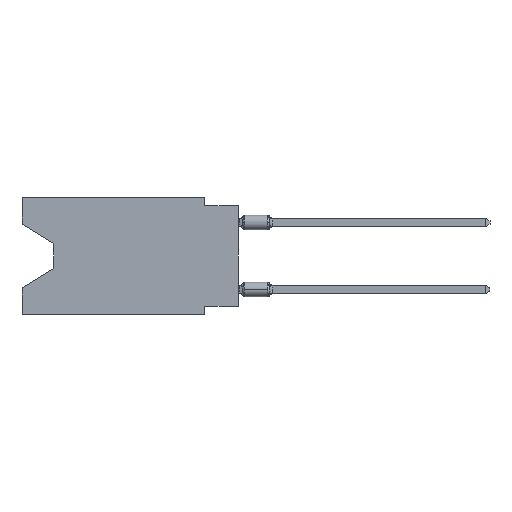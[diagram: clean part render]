
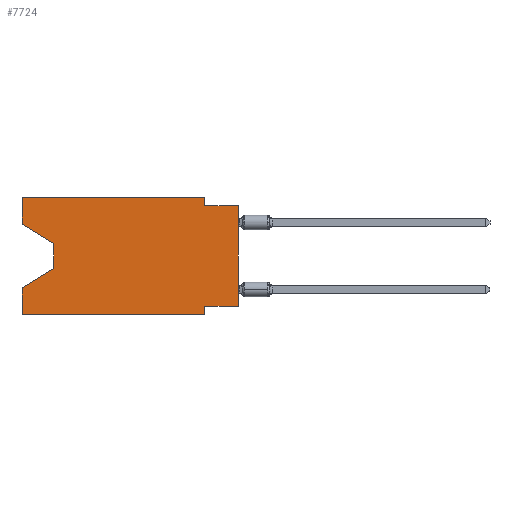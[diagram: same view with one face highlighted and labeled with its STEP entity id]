
A CAD part, left-side view. The second image highlights one B-rep face of the part: STEP entity #7724.
In plain terms, the highlighted planar face has unit normal (-1, 0, 0).
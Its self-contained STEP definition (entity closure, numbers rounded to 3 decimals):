
#244 = CARTESIAN_POINT ( 'NONE',  ( 0., 16.383, -6.852 ) ) ;
#472 = LINE ( 'NONE', #6832, #9910 ) ;
#887 = EDGE_CURVE ( 'NONE', #10630, #5363, #9956, .T. ) ;
#912 = CARTESIAN_POINT ( 'NONE',  ( 0., 0., -8.255 ) ) ;
#1674 = VECTOR ( 'NONE', #8993, 1000. ) ;
#1767 = CARTESIAN_POINT ( 'NONE',  ( 0., 2.54, -0.635 ) ) ;
#2021 = VERTEX_POINT ( 'NONE', #244 ) ;
#2134 = VECTOR ( 'NONE', #11825, 1000. ) ;
#2153 = DIRECTION ( 'NONE',  ( 0., 0., -1. ) ) ;
#2338 = VECTOR ( 'NONE', #5939, 1000. ) ;
#2572 = VERTEX_POINT ( 'NONE', #5486 ) ;
#2613 = LINE ( 'NONE', #3435, #10290 ) ;
#2792 = CARTESIAN_POINT ( 'NONE',  ( 0., 16.383, 0. ) ) ;
#2811 = CARTESIAN_POINT ( 'NONE',  ( 0., 0., -0.635 ) ) ;
#2906 = EDGE_CURVE ( 'NONE', #12319, #4956, #472, .T. ) ;
#2927 = CARTESIAN_POINT ( 'NONE',  ( 0., 13.97, -5.385 ) ) ;
#2950 = ORIENTED_EDGE ( 'NONE', *, *, #9825, .F. ) ;
#3041 = EDGE_CURVE ( 'NONE', #6452, #4927, #5234, .T. ) ;
#3043 = VERTEX_POINT ( 'NONE', #12381 ) ;
#3181 = AXIS2_PLACEMENT_3D ( 'NONE', #10889, #10615, #6629 ) ;
#3210 = ORIENTED_EDGE ( 'NONE', *, *, #4926, .F. ) ;
#3435 = CARTESIAN_POINT ( 'NONE',  ( 0., 2.54, -8.89 ) ) ;
#3523 = VERTEX_POINT ( 'NONE', #2927 ) ;
#3691 = LINE ( 'NONE', #2792, #5850 ) ;
#3751 = DIRECTION ( 'NONE',  ( 0., 0., 1. ) ) ;
#3907 = LINE ( 'NONE', #8965, #9124 ) ;
#3994 = ORIENTED_EDGE ( 'NONE', *, *, #5633, .F. ) ;
#4243 = CARTESIAN_POINT ( 'NONE',  ( 0., 2.54, -8.255 ) ) ;
#4353 = FACE_OUTER_BOUND ( 'NONE', #4786, .T. ) ;
#4506 = ORIENTED_EDGE ( 'NONE', *, *, #9095, .F. ) ;
#4655 = CARTESIAN_POINT ( 'NONE',  ( 0., 16.383, -2.038 ) ) ;
#4670 = CARTESIAN_POINT ( 'NONE',  ( 0., 16.383, -8.89 ) ) ;
#4786 = EDGE_LOOP ( 'NONE', ( #4982, #11441, #11220, #3210, #11460, #9499, #10386, #10284, #5818, #4506, #3994, #2950 ) ) ;
#4926 = EDGE_CURVE ( 'NONE', #12319, #2021, #3907, .T. ) ;
#4927 = VERTEX_POINT ( 'NONE', #2811 ) ;
#4956 = VERTEX_POINT ( 'NONE', #8124 ) ;
#4982 = ORIENTED_EDGE ( 'NONE', *, *, #887, .T. ) ;
#4996 = VERTEX_POINT ( 'NONE', #1767 ) ;
#5032 = LINE ( 'NONE', #6970, #2338 ) ;
#5234 = LINE ( 'NONE', #6060, #5507 ) ;
#5328 = LINE ( 'NONE', #912, #6021 ) ;
#5363 = VERTEX_POINT ( 'NONE', #10170 ) ;
#5364 = CARTESIAN_POINT ( 'NONE',  ( 0., 0., -8.255 ) ) ;
#5466 = LINE ( 'NONE', #10485, #8954 ) ;
#5486 = CARTESIAN_POINT ( 'NONE',  ( 0., 16.383, 0. ) ) ;
#5507 = VECTOR ( 'NONE', #6197, 1000. ) ;
#5633 = EDGE_CURVE ( 'NONE', #2572, #3043, #7622, .T. ) ;
#5818 = ORIENTED_EDGE ( 'NONE', *, *, #8997, .F. ) ;
#5850 = VECTOR ( 'NONE', #3751, 1000. ) ;
#5939 = DIRECTION ( 'NONE',  ( 0., -1., 0. ) ) ;
#6021 = VECTOR ( 'NONE', #9536, 1000. ) ;
#6060 = CARTESIAN_POINT ( 'NONE',  ( 0., 0., 0. ) ) ;
#6099 = VECTOR ( 'NONE', #12518, 1000. ) ;
#6197 = DIRECTION ( 'NONE',  ( 0., 0., 1. ) ) ;
#6452 = VERTEX_POINT ( 'NONE', #5364 ) ;
#6453 = CARTESIAN_POINT ( 'NONE',  ( 0., 16.383, 0. ) ) ;
#6629 = DIRECTION ( 'NONE',  ( 0., 0., -1. ) ) ;
#6773 = VERTEX_POINT ( 'NONE', #4243 ) ;
#6832 = CARTESIAN_POINT ( 'NONE',  ( 0., 16.383, -8.89 ) ) ;
#6970 = CARTESIAN_POINT ( 'NONE',  ( 0., 0., -0.635 ) ) ;
#7448 = DIRECTION ( 'NONE',  ( 0., 0., -1. ) ) ;
#7592 = PLANE ( 'NONE',  #3181 ) ;
#7622 = LINE ( 'NONE', #6453, #2134 ) ;
#7724 = ADVANCED_FACE ( 'NONE', ( #4353 ), #7592, .F. ) ;
#8037 = VECTOR ( 'NONE', #7448, 1000. ) ;
#8124 = CARTESIAN_POINT ( 'NONE',  ( 0., 2.54, -8.89 ) ) ;
#8462 = CARTESIAN_POINT ( 'NONE',  ( 0., 13.97, -5.385 ) ) ;
#8789 = EDGE_CURVE ( 'NONE', #5363, #3523, #5466, .T. ) ;
#8954 = VECTOR ( 'NONE', #2153, 1000. ) ;
#8965 = CARTESIAN_POINT ( 'NONE',  ( 0., 16.383, 0. ) ) ;
#8993 = DIRECTION ( 'NONE',  ( 0., -0.855, -0.519 ) ) ;
#8997 = EDGE_CURVE ( 'NONE', #4996, #4927, #5032, .T. ) ;
#9022 = CARTESIAN_POINT ( 'NONE',  ( 0., 16.383, -2.038 ) ) ;
#9028 = DIRECTION ( 'NONE',  ( 0., -1., 0. ) ) ;
#9095 = EDGE_CURVE ( 'NONE', #3043, #4996, #10671, .T. ) ;
#9124 = VECTOR ( 'NONE', #12315, 1000. ) ;
#9499 = ORIENTED_EDGE ( 'NONE', *, *, #10525, .F. ) ;
#9511 = CARTESIAN_POINT ( 'NONE',  ( 0., 2.54, 0. ) ) ;
#9536 = DIRECTION ( 'NONE',  ( 0., 1., 0. ) ) ;
#9825 = EDGE_CURVE ( 'NONE', #10630, #2572, #3691, .T. ) ;
#9910 = VECTOR ( 'NONE', #9028, 1000. ) ;
#9956 = LINE ( 'NONE', #4655, #1674 ) ;
#10170 = CARTESIAN_POINT ( 'NONE',  ( 0., 13.97, -3.505 ) ) ;
#10284 = ORIENTED_EDGE ( 'NONE', *, *, #3041, .T. ) ;
#10290 = VECTOR ( 'NONE', #12055, 1000. ) ;
#10386 = ORIENTED_EDGE ( 'NONE', *, *, #12981, .F. ) ;
#10485 = CARTESIAN_POINT ( 'NONE',  ( 0., 13.97, -3.505 ) ) ;
#10525 = EDGE_CURVE ( 'NONE', #6773, #4956, #2613, .T. ) ;
#10615 = DIRECTION ( 'NONE',  ( 1., 0., 0. ) ) ;
#10630 = VERTEX_POINT ( 'NONE', #9022 ) ;
#10671 = LINE ( 'NONE', #9511, #8037 ) ;
#10756 = EDGE_CURVE ( 'NONE', #3523, #2021, #13567, .T. ) ;
#10889 = CARTESIAN_POINT ( 'NONE',  ( 0., 16.383, 0. ) ) ;
#11220 = ORIENTED_EDGE ( 'NONE', *, *, #10756, .T. ) ;
#11441 = ORIENTED_EDGE ( 'NONE', *, *, #8789, .T. ) ;
#11460 = ORIENTED_EDGE ( 'NONE', *, *, #2906, .T. ) ;
#11825 = DIRECTION ( 'NONE',  ( 0., -1., 0. ) ) ;
#12055 = DIRECTION ( 'NONE',  ( 0., 0., -1. ) ) ;
#12315 = DIRECTION ( 'NONE',  ( 0., 0., 1. ) ) ;
#12319 = VERTEX_POINT ( 'NONE', #4670 ) ;
#12381 = CARTESIAN_POINT ( 'NONE',  ( 0., 2.54, 0. ) ) ;
#12518 = DIRECTION ( 'NONE',  ( 0., 0.855, -0.519 ) ) ;
#12981 = EDGE_CURVE ( 'NONE', #6452, #6773, #5328, .T. ) ;
#13567 = LINE ( 'NONE', #8462, #6099 ) ;
